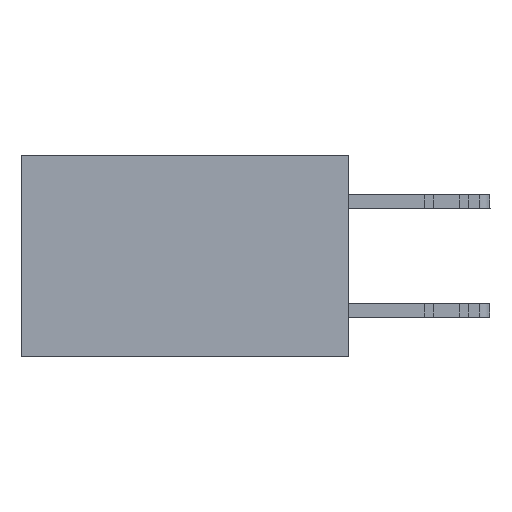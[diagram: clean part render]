
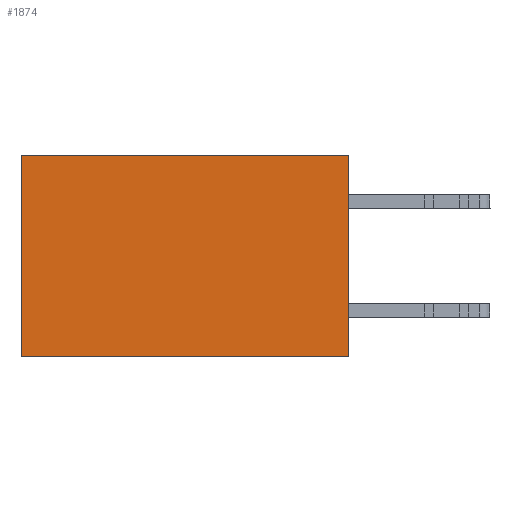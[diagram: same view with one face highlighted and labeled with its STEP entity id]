
A CAD part, left-side view. The second image highlights one B-rep face of the part: STEP entity #1874.
In plain terms, the highlighted planar face has unit normal (-1, 0, 0).
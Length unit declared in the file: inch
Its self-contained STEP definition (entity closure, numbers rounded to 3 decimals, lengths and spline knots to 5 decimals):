
#114 = LINE ( 'NONE', #17199, #22690 ) ;
#1547 = ORIENTED_EDGE ( 'NONE', *, *, #14931, .F. ) ;
#1643 = EDGE_LOOP ( 'NONE', ( #15723, #1547, #20920, #25045 ) ) ;
#1874 = ADVANCED_FACE ( 'NONE', ( #6345 ), #22727, .F. ) ;
#3234 = DIRECTION ( 'NONE',  ( 0., 0., -1. ) ) ;
#3282 = DIRECTION ( 'NONE',  ( 0., 1., 0. ) ) ;
#4948 = DIRECTION ( 'NONE',  ( 0., 0., -1. ) ) ;
#5736 = VERTEX_POINT ( 'NONE', #8067 ) ;
#6345 = FACE_OUTER_BOUND ( 'NONE', #1643, .T. ) ;
#7806 = CARTESIAN_POINT ( 'NONE',  ( 0.298, 0., 0. ) ) ;
#8067 = CARTESIAN_POINT ( 'NONE',  ( 0.298, 0.6, -0.37 ) ) ;
#9446 = VERTEX_POINT ( 'NONE', #25430 ) ;
#10094 = VERTEX_POINT ( 'NONE', #25697 ) ;
#11375 = VERTEX_POINT ( 'NONE', #25749 ) ;
#12277 = DIRECTION ( 'NONE',  ( 0., 0., -1. ) ) ;
#12493 = CARTESIAN_POINT ( 'NONE',  ( 0.298, 0.6, 0. ) ) ;
#12832 = EDGE_CURVE ( 'NONE', #10094, #11375, #114, .T. ) ;
#13137 = AXIS2_PLACEMENT_3D ( 'NONE', #7806, #27438, #3234 ) ;
#14121 = DIRECTION ( 'NONE',  ( 0., 1., 0. ) ) ;
#14931 = EDGE_CURVE ( 'NONE', #11375, #5736, #18734, .T. ) ;
#15723 = ORIENTED_EDGE ( 'NONE', *, *, #19480, .T. ) ;
#16428 = VECTOR ( 'NONE', #14121, 39.37008 ) ;
#17199 = CARTESIAN_POINT ( 'NONE',  ( 0.298, 0., 0. ) ) ;
#18734 = LINE ( 'NONE', #31499, #16428 ) ;
#19480 = EDGE_CURVE ( 'NONE', #9446, #5736, #26948, .T. ) ;
#20920 = ORIENTED_EDGE ( 'NONE', *, *, #12832, .F. ) ;
#22363 = VECTOR ( 'NONE', #12277, 39.37008 ) ;
#22690 = VECTOR ( 'NONE', #4948, 39.37008 ) ;
#22727 = PLANE ( 'NONE',  #13137 ) ;
#22898 = CARTESIAN_POINT ( 'NONE',  ( 0.298, 0., 0. ) ) ;
#24858 = VECTOR ( 'NONE', #3282, 39.37008 ) ;
#24994 = EDGE_CURVE ( 'NONE', #10094, #9446, #31324, .T. ) ;
#25045 = ORIENTED_EDGE ( 'NONE', *, *, #24994, .T. ) ;
#25430 = CARTESIAN_POINT ( 'NONE',  ( 0.298, 0.6, 0. ) ) ;
#25697 = CARTESIAN_POINT ( 'NONE',  ( 0.298, 0., 0. ) ) ;
#25749 = CARTESIAN_POINT ( 'NONE',  ( 0.298, 0., -0.37 ) ) ;
#26948 = LINE ( 'NONE', #12493, #22363 ) ;
#27438 = DIRECTION ( 'NONE',  ( 1., 0., 0. ) ) ;
#31324 = LINE ( 'NONE', #22898, #24858 ) ;
#31499 = CARTESIAN_POINT ( 'NONE',  ( 0.298, 0., -0.37 ) ) ;
